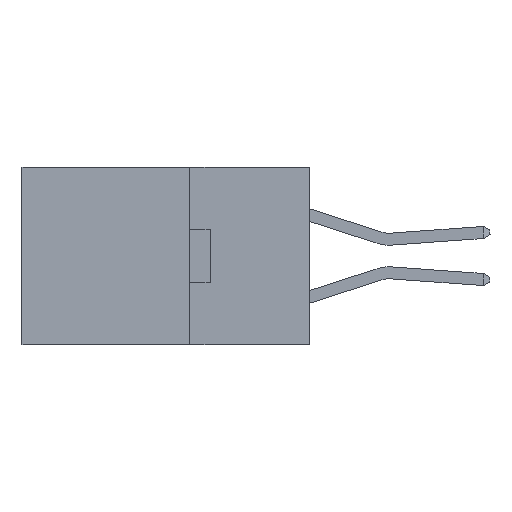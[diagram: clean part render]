
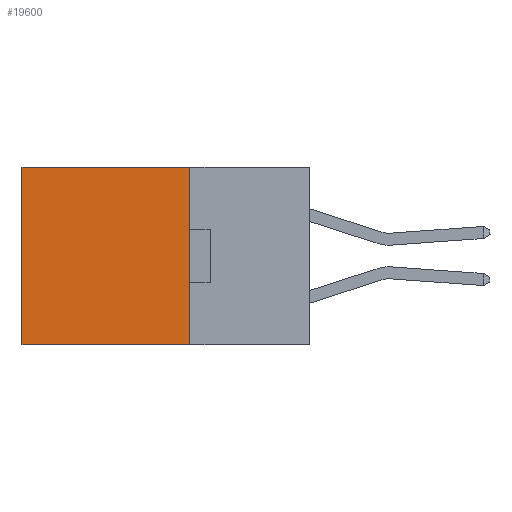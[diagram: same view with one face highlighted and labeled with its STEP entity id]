
A CAD part, left-side view. The second image highlights one B-rep face of the part: STEP entity #19600.
In plain terms, the highlighted planar face has unit normal (-1, 0, 0).
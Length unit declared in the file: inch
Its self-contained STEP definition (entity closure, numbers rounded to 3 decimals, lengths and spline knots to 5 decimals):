
#482 = CARTESIAN_POINT ( 'NONE',  ( 0.2615, 0.25, 0. ) ) ;
#2823 = DIRECTION ( 'NONE',  ( 0., 0., -1. ) ) ;
#3085 = CARTESIAN_POINT ( 'NONE',  ( 0.2615, 0.6, 0. ) ) ;
#3558 = CARTESIAN_POINT ( 'NONE',  ( 0.2615, 0.6, -0.37 ) ) ;
#4375 = VERTEX_POINT ( 'NONE', #3085 ) ;
#4663 = PLANE ( 'NONE',  #22416 ) ;
#6379 = CARTESIAN_POINT ( 'NONE',  ( 0.2615, 0.25, -0.37 ) ) ;
#6512 = LINE ( 'NONE', #6379, #7182 ) ;
#6871 = ORIENTED_EDGE ( 'NONE', *, *, #26954, .T. ) ;
#7182 = VECTOR ( 'NONE', #13016, 39.37008 ) ;
#8196 = VERTEX_POINT ( 'NONE', #21209 ) ;
#8355 = EDGE_CURVE ( 'NONE', #4375, #21632, #16111, .T. ) ;
#8641 = LINE ( 'NONE', #15123, #11353 ) ;
#9803 = EDGE_CURVE ( 'NONE', #22390, #8196, #6512, .T. ) ;
#10867 = FACE_OUTER_BOUND ( 'NONE', #18640, .T. ) ;
#11269 = ORIENTED_EDGE ( 'NONE', *, *, #19864, .F. ) ;
#11353 = VECTOR ( 'NONE', #23713, 39.37008 ) ;
#12088 = ORIENTED_EDGE ( 'NONE', *, *, #8355, .T. ) ;
#13016 = DIRECTION ( 'NONE',  ( 0., 0., -1. ) ) ;
#14351 = VECTOR ( 'NONE', #23247, 39.37008 ) ;
#15123 = CARTESIAN_POINT ( 'NONE',  ( 0.2615, 0.25, 0. ) ) ;
#15651 = DIRECTION ( 'NONE',  ( 1., 0., 0. ) ) ;
#15920 = ORIENTED_EDGE ( 'NONE', *, *, #9803, .F. ) ;
#16111 = LINE ( 'NONE', #3558, #23398 ) ;
#18640 = EDGE_LOOP ( 'NONE', ( #12088, #11269, #15920, #6871 ) ) ;
#19469 = CARTESIAN_POINT ( 'NONE',  ( 0.2615, 0.25, -0.37 ) ) ;
#19600 = ADVANCED_FACE ( 'NONE', ( #10867 ), #4663, .F. ) ;
#19864 = EDGE_CURVE ( 'NONE', #8196, #21632, #20992, .T. ) ;
#20544 = CARTESIAN_POINT ( 'NONE',  ( 0.2615, 0.6, -0.37 ) ) ;
#20992 = LINE ( 'NONE', #21270, #14351 ) ;
#21209 = CARTESIAN_POINT ( 'NONE',  ( 0.2615, 0.25, -0.37 ) ) ;
#21270 = CARTESIAN_POINT ( 'NONE',  ( 0.2615, 0.25, -0.37 ) ) ;
#21632 = VERTEX_POINT ( 'NONE', #20544 ) ;
#22390 = VERTEX_POINT ( 'NONE', #482 ) ;
#22416 = AXIS2_PLACEMENT_3D ( 'NONE', #19469, #15651, #2823 ) ;
#23247 = DIRECTION ( 'NONE',  ( 0., 1., 0. ) ) ;
#23398 = VECTOR ( 'NONE', #24831, 39.37008 ) ;
#23713 = DIRECTION ( 'NONE',  ( 0., 1., 0. ) ) ;
#24831 = DIRECTION ( 'NONE',  ( 0., 0., -1. ) ) ;
#26954 = EDGE_CURVE ( 'NONE', #22390, #4375, #8641, .T. ) ;
